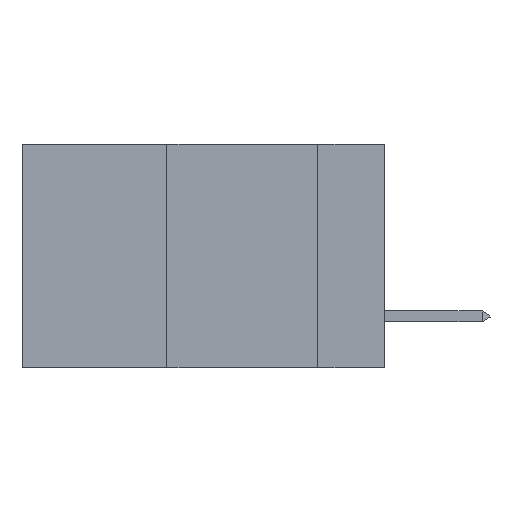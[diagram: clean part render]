
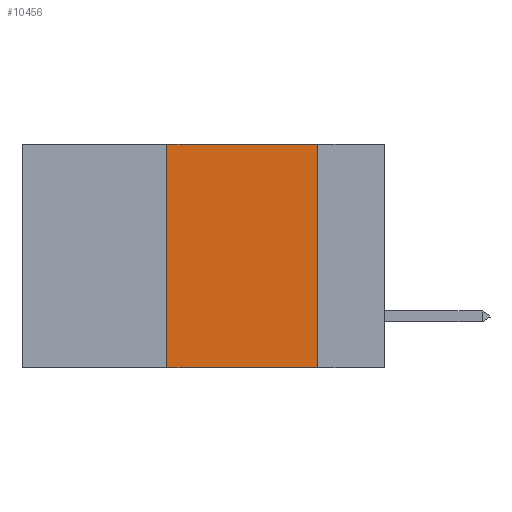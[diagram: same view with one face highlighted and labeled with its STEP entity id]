
A CAD part, left-side view. The second image highlights one B-rep face of the part: STEP entity #10456.
In plain terms, the highlighted planar face has unit normal (-1, 0, 0).
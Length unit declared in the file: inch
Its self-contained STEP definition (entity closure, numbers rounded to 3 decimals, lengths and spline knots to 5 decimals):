
#348 = VECTOR ( 'NONE', #15480, 39.37008 ) ;
#479 = CARTESIAN_POINT ( 'NONE',  ( 0., 0.36, -0.37 ) ) ;
#1269 = VECTOR ( 'NONE', #11062, 39.37008 ) ;
#1328 = CARTESIAN_POINT ( 'NONE',  ( 0., 0.11, 0. ) ) ;
#2360 = ORIENTED_EDGE ( 'NONE', *, *, #16778, .F. ) ;
#3412 = LINE ( 'NONE', #10811, #5117 ) ;
#5045 = ORIENTED_EDGE ( 'NONE', *, *, #21512, .F. ) ;
#5117 = VECTOR ( 'NONE', #16334, 39.37008 ) ;
#5466 = CARTESIAN_POINT ( 'NONE',  ( 0., 0.6, -0.37 ) ) ;
#6547 = CARTESIAN_POINT ( 'NONE',  ( 0., 0.6, 0. ) ) ;
#6654 = LINE ( 'NONE', #5466, #1269 ) ;
#6940 = EDGE_LOOP ( 'NONE', ( #17029, #5045, #2360, #14957 ) ) ;
#7196 = EDGE_CURVE ( 'NONE', #13899, #15271, #6654, .T. ) ;
#7284 = CARTESIAN_POINT ( 'NONE',  ( 0., 0.11, -0.37 ) ) ;
#8485 = DIRECTION ( 'NONE',  ( 0., 0., -1. ) ) ;
#9044 = LINE ( 'NONE', #1328, #348 ) ;
#9133 = FACE_OUTER_BOUND ( 'NONE', #6940, .T. ) ;
#9886 = CARTESIAN_POINT ( 'NONE',  ( 0., 0.36, 0. ) ) ;
#10126 = PLANE ( 'NONE',  #22157 ) ;
#10456 = ADVANCED_FACE ( 'NONE', ( #9133 ), #10126, .F. ) ;
#10811 = CARTESIAN_POINT ( 'NONE',  ( 0., 0.6, 0. ) ) ;
#11062 = DIRECTION ( 'NONE',  ( 0., -1., 0. ) ) ;
#11113 = VECTOR ( 'NONE', #15866, 39.37008 ) ;
#12819 = LINE ( 'NONE', #9886, #11113 ) ;
#13899 = VERTEX_POINT ( 'NONE', #479 ) ;
#14957 = ORIENTED_EDGE ( 'NONE', *, *, #7196, .T. ) ;
#15271 = VERTEX_POINT ( 'NONE', #7284 ) ;
#15480 = DIRECTION ( 'NONE',  ( 0., 0., -1. ) ) ;
#15824 = CARTESIAN_POINT ( 'NONE',  ( 0., 0.11, 0. ) ) ;
#15866 = DIRECTION ( 'NONE',  ( 0., 0., 1. ) ) ;
#15887 = EDGE_CURVE ( 'NONE', #21400, #15271, #9044, .T. ) ;
#16334 = DIRECTION ( 'NONE',  ( 0., -1., 0. ) ) ;
#16778 = EDGE_CURVE ( 'NONE', #13899, #23158, #12819, .T. ) ;
#17029 = ORIENTED_EDGE ( 'NONE', *, *, #15887, .F. ) ;
#17276 = CARTESIAN_POINT ( 'NONE',  ( 0., 0.36, 0. ) ) ;
#17321 = DIRECTION ( 'NONE',  ( 1., 0., 0. ) ) ;
#21400 = VERTEX_POINT ( 'NONE', #15824 ) ;
#21512 = EDGE_CURVE ( 'NONE', #23158, #21400, #3412, .T. ) ;
#22157 = AXIS2_PLACEMENT_3D ( 'NONE', #6547, #17321, #8485 ) ;
#23158 = VERTEX_POINT ( 'NONE', #17276 ) ;
